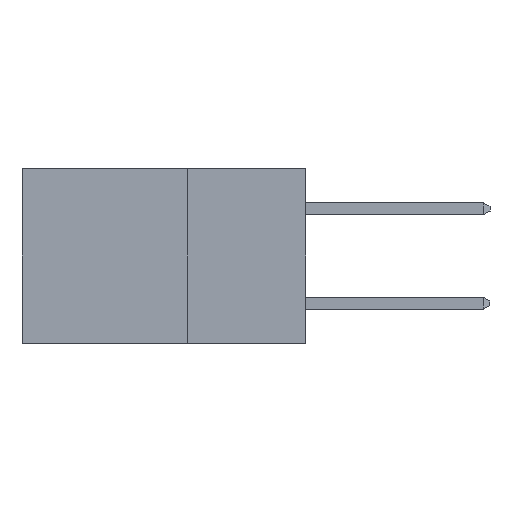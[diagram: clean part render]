
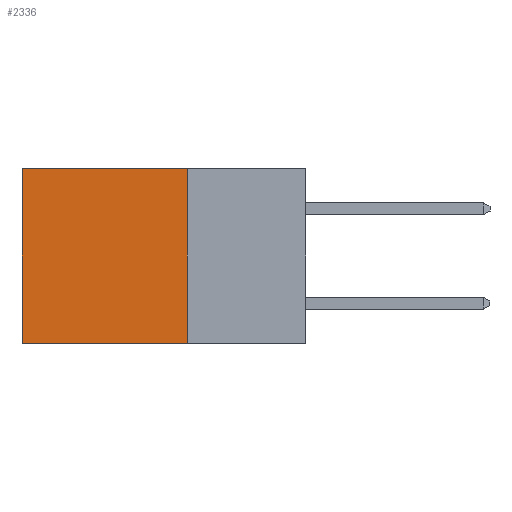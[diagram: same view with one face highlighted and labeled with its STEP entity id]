
A CAD part, left-side view. The second image highlights one B-rep face of the part: STEP entity #2336.
In plain terms, the highlighted planar face has unit normal (-1, 0, 0).
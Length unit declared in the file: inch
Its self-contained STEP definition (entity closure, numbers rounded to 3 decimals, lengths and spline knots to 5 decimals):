
#101 = VERTEX_POINT ( 'NONE', #2181 ) ;
#233 = DIRECTION ( 'NONE',  ( 0., 1., 0. ) ) ;
#313 = CARTESIAN_POINT ( 'NONE',  ( 0.298, 0.25, 0. ) ) ;
#1592 = VECTOR ( 'NONE', #3541, 39.37008 ) ;
#1637 = CARTESIAN_POINT ( 'NONE',  ( 0.298, 0.6, 0. ) ) ;
#2007 = FACE_OUTER_BOUND ( 'NONE', #14162, .T. ) ;
#2181 = CARTESIAN_POINT ( 'NONE',  ( 0.298, 0.25, -0.37 ) ) ;
#2336 = ADVANCED_FACE ( 'NONE', ( #2007 ), #18751, .F. ) ;
#3452 = VECTOR ( 'NONE', #3899, 39.37008 ) ;
#3468 = VERTEX_POINT ( 'NONE', #23534 ) ;
#3541 = DIRECTION ( 'NONE',  ( 0., 0., -1. ) ) ;
#3899 = DIRECTION ( 'NONE',  ( 0., 0., -1. ) ) ;
#4378 = VERTEX_POINT ( 'NONE', #20165 ) ;
#4942 = EDGE_CURVE ( 'NONE', #4378, #101, #8498, .T. ) ;
#5627 = VERTEX_POINT ( 'NONE', #10511 ) ;
#5799 = CARTESIAN_POINT ( 'NONE',  ( 0.298, 0.25, -0.37 ) ) ;
#6627 = ORIENTED_EDGE ( 'NONE', *, *, #7234, .T. ) ;
#6810 = VECTOR ( 'NONE', #7688, 39.37008 ) ;
#7234 = EDGE_CURVE ( 'NONE', #3468, #5627, #22830, .T. ) ;
#7688 = DIRECTION ( 'NONE',  ( 0., 1., 0. ) ) ;
#8498 = LINE ( 'NONE', #14332, #3452 ) ;
#10511 = CARTESIAN_POINT ( 'NONE',  ( 0.298, 0.6, -0.37 ) ) ;
#13942 = EDGE_CURVE ( 'NONE', #4378, #3468, #22123, .T. ) ;
#14162 = EDGE_LOOP ( 'NONE', ( #6627, #20389, #14750, #15477 ) ) ;
#14332 = CARTESIAN_POINT ( 'NONE',  ( 0.298, 0.25, 0. ) ) ;
#14750 = ORIENTED_EDGE ( 'NONE', *, *, #4942, .F. ) ;
#15477 = ORIENTED_EDGE ( 'NONE', *, *, #13942, .T. ) ;
#16702 = LINE ( 'NONE', #5799, #6810 ) ;
#17275 = VECTOR ( 'NONE', #233, 39.37008 ) ;
#17642 = DIRECTION ( 'NONE',  ( 1., 0., 0. ) ) ;
#17754 = DIRECTION ( 'NONE',  ( 0., 0., -1. ) ) ;
#18751 = PLANE ( 'NONE',  #20228 ) ;
#19797 = CARTESIAN_POINT ( 'NONE',  ( 0.298, 0.25, 0. ) ) ;
#20165 = CARTESIAN_POINT ( 'NONE',  ( 0.298, 0.25, 0. ) ) ;
#20228 = AXIS2_PLACEMENT_3D ( 'NONE', #19797, #17642, #17754 ) ;
#20389 = ORIENTED_EDGE ( 'NONE', *, *, #23049, .F. ) ;
#22123 = LINE ( 'NONE', #313, #17275 ) ;
#22830 = LINE ( 'NONE', #1637, #1592 ) ;
#23049 = EDGE_CURVE ( 'NONE', #101, #5627, #16702, .T. ) ;
#23534 = CARTESIAN_POINT ( 'NONE',  ( 0.298, 0.6, 0. ) ) ;
